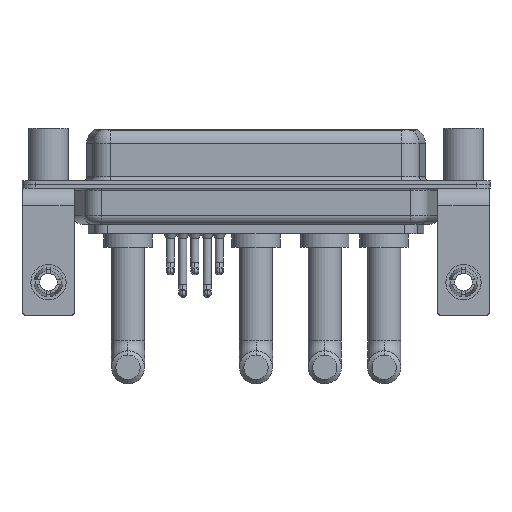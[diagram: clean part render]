
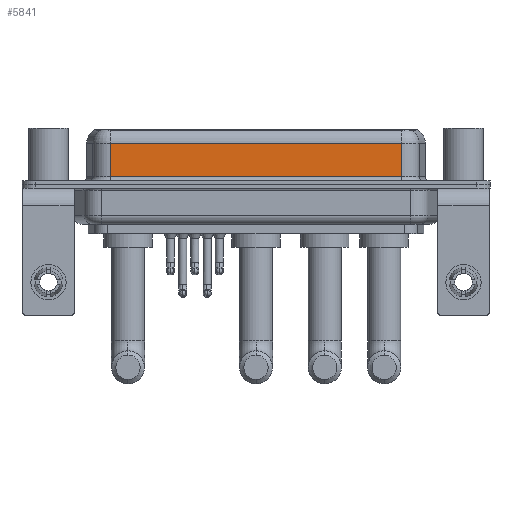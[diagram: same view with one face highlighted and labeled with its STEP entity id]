
A CAD part, front view. The second image highlights one B-rep face of the part: STEP entity #5841.
In plain terms, the highlighted planar face has unit normal (0, -1, 0).
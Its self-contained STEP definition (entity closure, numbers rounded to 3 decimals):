
#125 = VERTEX_POINT ( 'NONE', #15274 ) ;
#447 = CARTESIAN_POINT ( 'NONE',  ( 7.013, -3.95, 4.65 ) ) ;
#841 = ORIENTED_EDGE ( 'NONE', *, *, #15005, .T. ) ;
#1245 = PLANE ( 'NONE',  #1801 ) ;
#1349 = DIRECTION ( 'NONE',  ( 0., 1., 0. ) ) ;
#1801 = AXIS2_PLACEMENT_3D ( 'NONE', #7831, #1349, #14452 ) ;
#2363 = DIRECTION ( 'NONE',  ( 1., 0., 0. ) ) ;
#2801 = VECTOR ( 'NONE', #2363, 1000. ) ;
#3247 = EDGE_CURVE ( 'NONE', #12771, #125, #3326, .T. ) ;
#3326 = LINE ( 'NONE', #16534, #15256 ) ;
#3684 = CARTESIAN_POINT ( 'NONE',  ( 40.037, -3.95, 4.65 ) ) ;
#4440 = LINE ( 'NONE', #12571, #10785 ) ;
#5039 = ORIENTED_EDGE ( 'NONE', *, *, #21128, .F. ) ;
#5063 = CARTESIAN_POINT ( 'NONE',  ( 40.037, -3.95, 4.65 ) ) ;
#5266 = VERTEX_POINT ( 'NONE', #3684 ) ;
#5841 = ADVANCED_FACE ( 'NONE', ( #6094 ), #1245, .F. ) ;
#6094 = FACE_OUTER_BOUND ( 'NONE', #6263, .T. ) ;
#6263 = EDGE_LOOP ( 'NONE', ( #5039, #841, #13873, #18856 ) ) ;
#7473 = DIRECTION ( 'NONE',  ( 0., 0., -1. ) ) ;
#7831 = CARTESIAN_POINT ( 'NONE',  ( 40.037, -3.95, 6.4 ) ) ;
#9242 = VECTOR ( 'NONE', #18515, 1000. ) ;
#10288 = LINE ( 'NONE', #5063, #9242 ) ;
#10785 = VECTOR ( 'NONE', #7473, 1000. ) ;
#12571 = CARTESIAN_POINT ( 'NONE',  ( 40.037, -3.95, 6.4 ) ) ;
#12771 = VERTEX_POINT ( 'NONE', #447 ) ;
#13873 = ORIENTED_EDGE ( 'NONE', *, *, #3247, .T. ) ;
#14397 = VERTEX_POINT ( 'NONE', #20616 ) ;
#14452 = DIRECTION ( 'NONE',  ( 0., 0., 1. ) ) ;
#15005 = EDGE_CURVE ( 'NONE', #5266, #12771, #10288, .T. ) ;
#15256 = VECTOR ( 'NONE', #16210, 1000. ) ;
#15274 = CARTESIAN_POINT ( 'NONE',  ( 7.013, -3.95, 0.9 ) ) ;
#16210 = DIRECTION ( 'NONE',  ( 0., 0., -1. ) ) ;
#16534 = CARTESIAN_POINT ( 'NONE',  ( 7.013, -3.95, 6.4 ) ) ;
#17191 = CARTESIAN_POINT ( 'NONE',  ( 40.037, -3.95, 0.9 ) ) ;
#18515 = DIRECTION ( 'NONE',  ( -1., 0., 0. ) ) ;
#18856 = ORIENTED_EDGE ( 'NONE', *, *, #20283, .T. ) ;
#19655 = LINE ( 'NONE', #17191, #2801 ) ;
#20283 = EDGE_CURVE ( 'NONE', #125, #14397, #19655, .T. ) ;
#20616 = CARTESIAN_POINT ( 'NONE',  ( 40.037, -3.95, 0.9 ) ) ;
#21128 = EDGE_CURVE ( 'NONE', #5266, #14397, #4440, .T. ) ;
